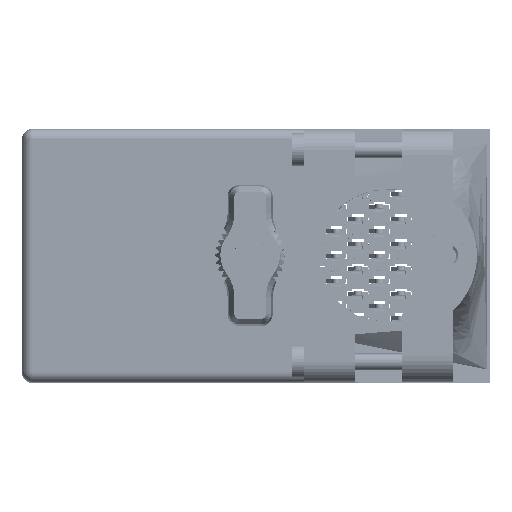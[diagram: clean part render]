
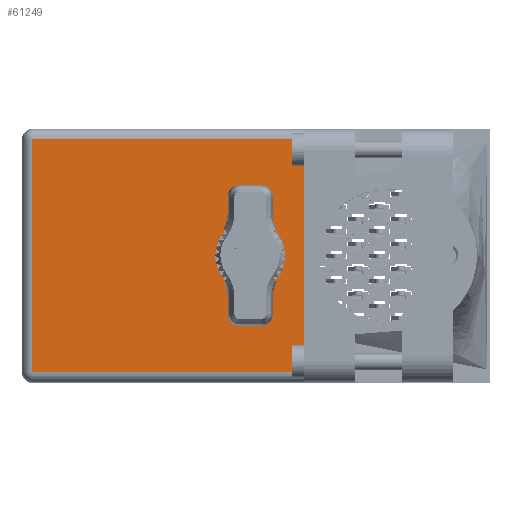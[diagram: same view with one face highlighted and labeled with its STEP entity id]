
A CAD part, top view. The second image highlights one B-rep face of the part: STEP entity #61249.
In plain terms, the highlighted face is planar.
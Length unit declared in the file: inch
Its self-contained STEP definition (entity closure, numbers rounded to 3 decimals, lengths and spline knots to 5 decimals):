
#2026 = ORIENTED_EDGE ( 'NONE', *, *, #114787, .T. ) ;
#3377 = DIRECTION ( 'NONE',  ( 0., 0., 1. ) ) ;
#8480 = CARTESIAN_POINT ( 'NONE',  ( 0., 1.93, 0. ) ) ;
#11330 = ORIENTED_EDGE ( 'NONE', *, *, #88445, .T. ) ;
#14971 = LINE ( 'NONE', #78597, #40196 ) ;
#19992 = DIRECTION ( 'NONE',  ( -1., 0., 0. ) ) ;
#20170 = VERTEX_POINT ( 'NONE', #113614 ) ;
#23617 = CARTESIAN_POINT ( 'NONE',  ( 0.3275, 1.93, -0.765 ) ) ;
#26509 = DIRECTION ( 'NONE',  ( 0., 1., 0. ) ) ;
#28294 = DIRECTION ( 'NONE',  ( 1., 0., 0. ) ) ;
#28901 = VERTEX_POINT ( 'NONE', #93263 ) ;
#29610 = VECTOR ( 'NONE', #104892, 39.37008 ) ;
#30093 = FACE_OUTER_BOUND ( 'NONE', #44917, .T. ) ;
#30300 = CARTESIAN_POINT ( 'NONE',  ( 0., 1.93, 0.17 ) ) ;
#32632 = CARTESIAN_POINT ( 'NONE',  ( -1.3155, 1.93, 0.703 ) ) ;
#32682 = ORIENTED_EDGE ( 'NONE', *, *, #107342, .F. ) ;
#33324 = CARTESIAN_POINT ( 'NONE',  ( -1.3155, 1.93, -0.765 ) ) ;
#40089 = VECTOR ( 'NONE', #28294, 39.37008 ) ;
#40196 = VECTOR ( 'NONE', #87628, 39.37008 ) ;
#44017 = CIRCLE ( 'NONE', #101422, 0.17 ) ;
#44917 = EDGE_LOOP ( 'NONE', ( #11330, #2026, #32682, #49469 ) ) ;
#46535 = DIRECTION ( 'NONE',  ( 0., 1., 0. ) ) ;
#49469 = ORIENTED_EDGE ( 'NONE', *, *, #84099, .T. ) ;
#50604 = EDGE_CURVE ( 'NONE', #66725, #62653, #81073, .T. ) ;
#54783 = CARTESIAN_POINT ( 'NONE',  ( -1.3775, 1.93, -0.765 ) ) ;
#56172 = EDGE_LOOP ( 'NONE', ( #77595, #60108 ) ) ;
#59642 = LINE ( 'NONE', #108036, #40089 ) ;
#60108 = ORIENTED_EDGE ( 'NONE', *, *, #50604, .F. ) ;
#60324 = DIRECTION ( 'NONE',  ( 0., 0., 1. ) ) ;
#61249 = ADVANCED_FACE ( 'NONE', ( #30093, #99959 ), #80933, .T. ) ;
#61659 = DIRECTION ( 'NONE',  ( 0., 0., 1. ) ) ;
#62653 = VERTEX_POINT ( 'NONE', #30300 ) ;
#65152 = VECTOR ( 'NONE', #60324, 39.37008 ) ;
#66725 = VERTEX_POINT ( 'NONE', #115758 ) ;
#73568 = LINE ( 'NONE', #23617, #65152 ) ;
#74901 = CARTESIAN_POINT ( 'NONE',  ( 0., 1.93, 0. ) ) ;
#75859 = VERTEX_POINT ( 'NONE', #106657 ) ;
#77595 = ORIENTED_EDGE ( 'NONE', *, *, #85442, .F. ) ;
#78597 = CARTESIAN_POINT ( 'NONE',  ( -1.3775, 1.93, -0.703 ) ) ;
#80933 = PLANE ( 'NONE',  #89903 ) ;
#81073 = CIRCLE ( 'NONE', #115984, 0.17 ) ;
#84099 = EDGE_CURVE ( 'NONE', #20170, #75859, #14971, .T. ) ;
#85442 = EDGE_CURVE ( 'NONE', #62653, #66725, #44017, .T. ) ;
#87628 = DIRECTION ( 'NONE',  ( -1., 0., 0. ) ) ;
#88445 = EDGE_CURVE ( 'NONE', #75859, #105996, #112067, .T. ) ;
#89903 = AXIS2_PLACEMENT_3D ( 'NONE', #54783, #46535, #19992 ) ;
#93263 = CARTESIAN_POINT ( 'NONE',  ( 0.3275, 1.93, 0.703 ) ) ;
#99959 = FACE_BOUND ( 'NONE', #56172, .T. ) ;
#100760 = DIRECTION ( 'NONE',  ( 0., 1., 0. ) ) ;
#101422 = AXIS2_PLACEMENT_3D ( 'NONE', #8480, #26509, #61659 ) ;
#104892 = DIRECTION ( 'NONE',  ( 0., 0., 1. ) ) ;
#105996 = VERTEX_POINT ( 'NONE', #32632 ) ;
#106657 = CARTESIAN_POINT ( 'NONE',  ( -1.3155, 1.93, -0.703 ) ) ;
#107342 = EDGE_CURVE ( 'NONE', #20170, #28901, #73568, .T. ) ;
#108036 = CARTESIAN_POINT ( 'NONE',  ( 0.3275, 1.93, 0.703 ) ) ;
#112067 = LINE ( 'NONE', #33324, #29610 ) ;
#113614 = CARTESIAN_POINT ( 'NONE',  ( 0.3275, 1.93, -0.703 ) ) ;
#114787 = EDGE_CURVE ( 'NONE', #105996, #28901, #59642, .T. ) ;
#115758 = CARTESIAN_POINT ( 'NONE',  ( 0., 1.93, -0.17 ) ) ;
#115984 = AXIS2_PLACEMENT_3D ( 'NONE', #74901, #100760, #3377 ) ;
